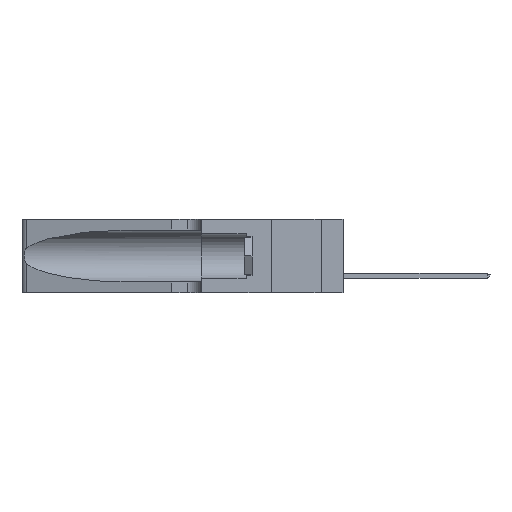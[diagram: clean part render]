
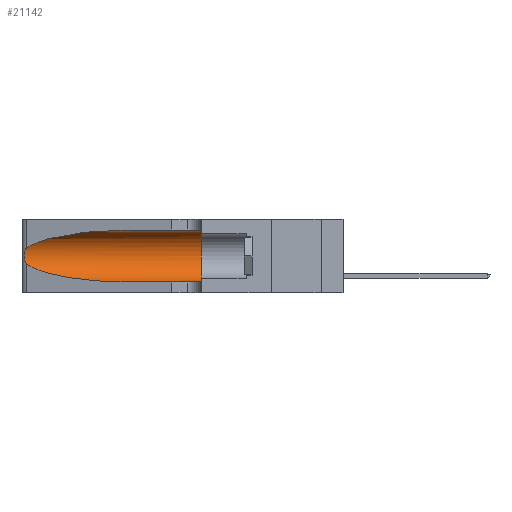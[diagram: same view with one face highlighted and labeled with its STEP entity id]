
A CAD part, left-side view. The second image highlights one B-rep face of the part: STEP entity #21142.
In plain terms, the highlighted cylindrical face has radius 3.308 mm (diameter 6.617 mm), a partial arc.
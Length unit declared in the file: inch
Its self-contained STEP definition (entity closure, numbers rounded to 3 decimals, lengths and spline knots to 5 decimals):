
#57 = FACE_OUTER_BOUND ( 'NONE', #36487, .T. ) ;
#256 = ORIENTED_EDGE ( 'NONE', *, *, #25905, .T. ) ;
#1775 = CARTESIAN_POINT ( 'NONE',  ( 0.2373, 1.15595, 0.28018 ) ) ;
#2338 = VERTEX_POINT ( 'NONE', #16111 ) ;
#2500 = CARTESIAN_POINT ( 'NONE',  ( 0.18966, 0.96281, 0.05475 ) ) ;
#3018 = LINE ( 'NONE', #12604, #21675 ) ;
#4489 = CARTESIAN_POINT ( 'NONE',  ( 0.25854, 1.2359, 0.20912 ) ) ;
#5175 = EDGE_CURVE ( 'NONE', #46921, #2338, #22082, .T. ) ;
#5857 = ORIENTED_EDGE ( 'NONE', *, *, #31790, .F. ) ;
#5999 = CARTESIAN_POINT ( 'NONE',  ( 0.25487, 1.22718, 0.14631 ) ) ;
#6106 = VERTEX_POINT ( 'NONE', #35567 ) ;
#8734 = EDGE_CURVE ( 'NONE', #46035, #6106, #42339, .T. ) ;
#10010 = CIRCLE ( 'NONE', #37075, 0.13025 ) ;
#12215 = CARTESIAN_POINT ( 'NONE',  ( 0.25555, 1.22994, 0.2215 ) ) ;
#12541 = DIRECTION ( 'NONE',  ( 0., -1., 0. ) ) ;
#12558 = CARTESIAN_POINT ( 'NONE',  ( 0.25789, 1.23486, 0.15765 ) ) ;
#12604 = CARTESIAN_POINT ( 'NONE',  ( 0.1305, 1.61858, 0.05475 ) ) ;
#14585 = DIRECTION ( 'NONE',  ( 0., 0., -1. ) ) ;
#16111 = CARTESIAN_POINT ( 'NONE',  ( 0.1305, 0.72297, 0.05475 ) ) ;
#16299 = VERTEX_POINT ( 'NONE', #29021 ) ;
#16566 = CARTESIAN_POINT ( 'NONE',  ( 0.26017, 1.23833, 0.17102 ) ) ;
#16623 = DIRECTION ( 'NONE',  ( 0., -1., 0. ) ) ;
#20067 = CARTESIAN_POINT ( 'NONE',  ( 0.25555, 1.22993, 0.14849 ) ) ;
#20122 = DIRECTION ( 'NONE',  ( 0., -1., 0. ) ) ;
#20220 = CARTESIAN_POINT ( 'NONE',  ( 0.26075, 1.23896, 0.19203 ) ) ;
#21142 = ADVANCED_FACE ( 'NONE', ( #57 ), #51453, .F. ) ;
#21675 = VECTOR ( 'NONE', #16623, 39.37008 ) ;
#21804 = DIRECTION ( 'NONE',  ( 0., 0., 1. ) ) ;
#22082 =( BOUNDED_CURVE ( )  B_SPLINE_CURVE ( 3, ( #5999, #37587, #2500, #30461 ),
 .UNSPECIFIED., .F., .F. ) 
 B_SPLINE_CURVE_WITH_KNOTS ( ( 4, 4 ),
 ( 3.44316, 4.71239 ),
 .UNSPECIFIED. ) 
 CURVE ( )  GEOMETRIC_REPRESENTATION_ITEM ( )  RATIONAL_B_SPLINE_CURVE ( ( 1., 0.87, 0.87, 1. ) ) 
 REPRESENTATION_ITEM ( '' )  );
#23351 = LINE ( 'NONE', #44084, #44623 ) ;
#23864 = CARTESIAN_POINT ( 'NONE',  ( 0.26075, 1.23896, 0.178 ) ) ;
#25905 = EDGE_CURVE ( 'NONE', #6106, #46921, #34616, .T. ) ;
#28797 = CARTESIAN_POINT ( 'NONE',  ( 0.1305, 0.72297, 0.31525 ) ) ;
#29021 = CARTESIAN_POINT ( 'NONE',  ( 0.1305, 0.35, 0.31525 ) ) ;
#30461 = CARTESIAN_POINT ( 'NONE',  ( 0.1305, 0.72297, 0.05475 ) ) ;
#31790 = EDGE_CURVE ( 'NONE', #46035, #16299, #23351, .T. ) ;
#33762 = CARTESIAN_POINT ( 'NONE',  ( 0.25487, 1.22718, 0.22369 ) ) ;
#33952 = EDGE_CURVE ( 'NONE', #16299, #50552, #10010, .T. ) ;
#34495 = CARTESIAN_POINT ( 'NONE',  ( 0.18966, 0.96281, 0.31525 ) ) ;
#34616 = B_SPLINE_CURVE_WITH_KNOTS ( 'NONE', 3,
 ( #33762, #12215, #40331, #44183, #4489, #39878, #20220, #23864, #16566, #48247, #12558, #44026, #20067, #40501 ),
 .UNSPECIFIED., .F., .F.,
 ( 4, 2, 2, 2, 2, 2, 4 ),
 ( 0., 0.00027, 0.00053, 0.00107, 0.0016, 0.00187, 0.00214 ),
 .UNSPECIFIED. ) ;
#35567 = CARTESIAN_POINT ( 'NONE',  ( 0.25487, 1.22718, 0.22369 ) ) ;
#36487 = EDGE_LOOP ( 'NONE', ( #49492, #256, #43710, #41705, #46873, #5857 ) ) ;
#37075 = AXIS2_PLACEMENT_3D ( 'NONE', #45814, #45470, #21804 ) ;
#37587 = CARTESIAN_POINT ( 'NONE',  ( 0.2373, 1.15595, 0.08982 ) ) ;
#38220 = CARTESIAN_POINT ( 'NONE',  ( 0.25487, 1.22718, 0.14631 ) ) ;
#39878 = CARTESIAN_POINT ( 'NONE',  ( 0.26018, 1.23835, 0.19895 ) ) ;
#40331 = CARTESIAN_POINT ( 'NONE',  ( 0.25639, 1.23184, 0.21858 ) ) ;
#40501 = CARTESIAN_POINT ( 'NONE',  ( 0.25487, 1.22718, 0.14631 ) ) ;
#41671 = CARTESIAN_POINT ( 'NONE',  ( 0.1305, 0.72297, 0.31525 ) ) ;
#41705 = ORIENTED_EDGE ( 'NONE', *, *, #43110, .T. ) ;
#41770 = AXIS2_PLACEMENT_3D ( 'NONE', #44990, #12541, #14585 ) ;
#42339 =( BOUNDED_CURVE ( )  B_SPLINE_CURVE ( 3, ( #41671, #34495, #1775, #42936 ),
 .UNSPECIFIED., .F., .T. ) 
 B_SPLINE_CURVE_WITH_KNOTS ( ( 4, 4 ),
 ( 1.5708, 2.84003 ),
 .UNSPECIFIED. ) 
 CURVE ( )  GEOMETRIC_REPRESENTATION_ITEM ( )  RATIONAL_B_SPLINE_CURVE ( ( 1., 0.87, 0.87, 1. ) ) 
 REPRESENTATION_ITEM ( '' )  );
#42936 = CARTESIAN_POINT ( 'NONE',  ( 0.25487, 1.22718, 0.22369 ) ) ;
#43110 = EDGE_CURVE ( 'NONE', #2338, #50552, #3018, .T. ) ;
#43710 = ORIENTED_EDGE ( 'NONE', *, *, #5175, .T. ) ;
#44026 = CARTESIAN_POINT ( 'NONE',  ( 0.25639, 1.23186, 0.15144 ) ) ;
#44084 = CARTESIAN_POINT ( 'NONE',  ( 0.1305, 1.61858, 0.31525 ) ) ;
#44183 = CARTESIAN_POINT ( 'NONE',  ( 0.25787, 1.23484, 0.2124 ) ) ;
#44623 = VECTOR ( 'NONE', #20122, 39.37008 ) ;
#44990 = CARTESIAN_POINT ( 'NONE',  ( 0.1305, 1.61858, 0.185 ) ) ;
#45470 = DIRECTION ( 'NONE',  ( 0., 1., 0. ) ) ;
#45492 = CARTESIAN_POINT ( 'NONE',  ( 0.1305, 0.35, 0.05475 ) ) ;
#45814 = CARTESIAN_POINT ( 'NONE',  ( 0.1305, 0.35, 0.185 ) ) ;
#46035 = VERTEX_POINT ( 'NONE', #28797 ) ;
#46873 = ORIENTED_EDGE ( 'NONE', *, *, #33952, .F. ) ;
#46921 = VERTEX_POINT ( 'NONE', #38220 ) ;
#48247 = CARTESIAN_POINT ( 'NONE',  ( 0.25856, 1.23593, 0.16098 ) ) ;
#49492 = ORIENTED_EDGE ( 'NONE', *, *, #8734, .T. ) ;
#50552 = VERTEX_POINT ( 'NONE', #45492 ) ;
#51453 = CYLINDRICAL_SURFACE ( 'NONE', #41770, 0.13025 ) ;
